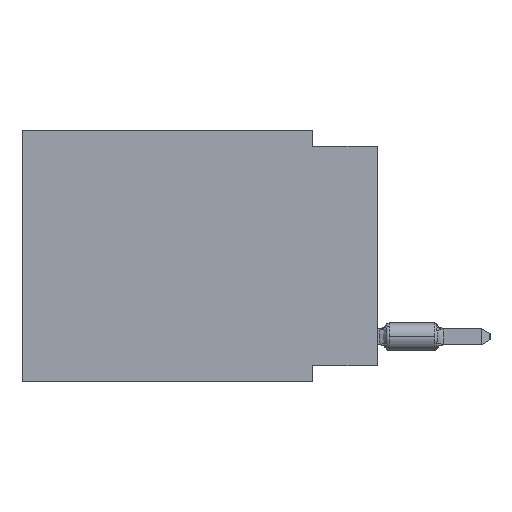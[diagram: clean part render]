
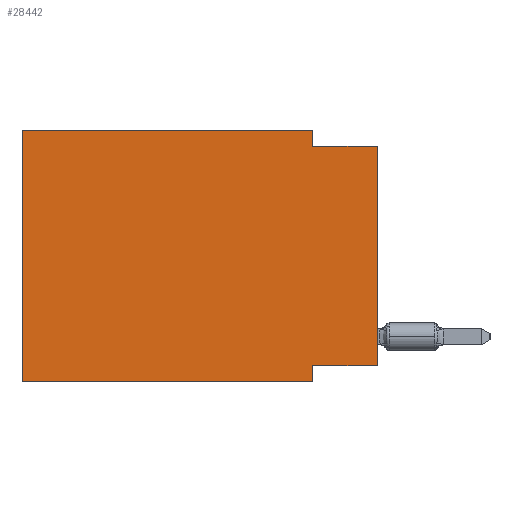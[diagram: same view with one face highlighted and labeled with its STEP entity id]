
A CAD part, left-side view. The second image highlights one B-rep face of the part: STEP entity #28442.
In plain terms, the highlighted planar face has unit normal (-1, 0, 0).
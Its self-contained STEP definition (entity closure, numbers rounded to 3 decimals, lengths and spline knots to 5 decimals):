
#246 = ORIENTED_EDGE ( 'NONE', *, *, #40371, .F. ) ;
#853 = DIRECTION ( 'NONE',  ( 0., -1., 0. ) ) ;
#866 = VERTEX_POINT ( 'NONE', #21386 ) ;
#4461 = LINE ( 'NONE', #12901, #59141 ) ;
#5445 = CARTESIAN_POINT ( 'NONE',  ( 0., 0.55, 0. ) ) ;
#7250 = CARTESIAN_POINT ( 'NONE',  ( 0., 0.1, -0.39 ) ) ;
#7344 = DIRECTION ( 'NONE',  ( 0., -1., 0. ) ) ;
#8345 = VERTEX_POINT ( 'NONE', #37222 ) ;
#8812 = EDGE_CURVE ( 'NONE', #8345, #47510, #38038, .T. ) ;
#9786 = DIRECTION ( 'NONE',  ( 0., 0., 1. ) ) ;
#10317 = VECTOR ( 'NONE', #9786, 39.37008 ) ;
#11092 = ORIENTED_EDGE ( 'NONE', *, *, #44853, .F. ) ;
#11502 = LINE ( 'NONE', #44207, #32913 ) ;
#12847 = VECTOR ( 'NONE', #15219, 39.37008 ) ;
#12901 = CARTESIAN_POINT ( 'NONE',  ( 0., 0.1, -0.39 ) ) ;
#13171 = ORIENTED_EDGE ( 'NONE', *, *, #41243, .F. ) ;
#13250 = VECTOR ( 'NONE', #52346, 39.37008 ) ;
#13631 = VECTOR ( 'NONE', #40186, 39.37008 ) ;
#14652 = CARTESIAN_POINT ( 'NONE',  ( 0., 0.1, 0. ) ) ;
#15219 = DIRECTION ( 'NONE',  ( 0., -1., 0. ) ) ;
#15557 = EDGE_LOOP ( 'NONE', ( #50107, #246, #11092, #27466, #23908, #59006, #13171, #59158 ) ) ;
#17220 = LINE ( 'NONE', #54148, #37976 ) ;
#20339 = CARTESIAN_POINT ( 'NONE',  ( 0., 0., -0.365 ) ) ;
#21386 = CARTESIAN_POINT ( 'NONE',  ( 0., 0.1, -0.025 ) ) ;
#23020 = PLANE ( 'NONE',  #30125 ) ;
#23908 = ORIENTED_EDGE ( 'NONE', *, *, #44401, .F. ) ;
#26352 = CARTESIAN_POINT ( 'NONE',  ( 0., 0., 0. ) ) ;
#27466 = ORIENTED_EDGE ( 'NONE', *, *, #31068, .F. ) ;
#27755 = VERTEX_POINT ( 'NONE', #30049 ) ;
#28442 = ADVANCED_FACE ( 'NONE', ( #37157 ), #23020, .F. ) ;
#29666 = CARTESIAN_POINT ( 'NONE',  ( 0., 0., -0.025 ) ) ;
#30049 = CARTESIAN_POINT ( 'NONE',  ( 0., 0.1, -0.365 ) ) ;
#30099 = DIRECTION ( 'NONE',  ( 0., 1., 0. ) ) ;
#30125 = AXIS2_PLACEMENT_3D ( 'NONE', #55450, #41665, #41961 ) ;
#31068 = EDGE_CURVE ( 'NONE', #32245, #34692, #33575, .T. ) ;
#31189 = VECTOR ( 'NONE', #853, 39.37008 ) ;
#31235 = VERTEX_POINT ( 'NONE', #29666 ) ;
#32245 = VERTEX_POINT ( 'NONE', #5445 ) ;
#32891 = DIRECTION ( 'NONE',  ( 0., 0., -1. ) ) ;
#32913 = VECTOR ( 'NONE', #30099, 39.37008 ) ;
#33575 = LINE ( 'NONE', #42006, #31189 ) ;
#33721 = CARTESIAN_POINT ( 'NONE',  ( 0., 0.1, 0. ) ) ;
#34692 = VERTEX_POINT ( 'NONE', #14652 ) ;
#36417 = VERTEX_POINT ( 'NONE', #20339 ) ;
#36528 = CARTESIAN_POINT ( 'NONE',  ( 0., 0.55, 0. ) ) ;
#37157 = FACE_OUTER_BOUND ( 'NONE', #15557, .T. ) ;
#37222 = CARTESIAN_POINT ( 'NONE',  ( 0., 0.55, -0.39 ) ) ;
#37240 = EDGE_CURVE ( 'NONE', #36417, #27755, #11502, .T. ) ;
#37941 = LINE ( 'NONE', #33721, #13250 ) ;
#37976 = VECTOR ( 'NONE', #7344, 39.37008 ) ;
#38038 = LINE ( 'NONE', #56344, #12847 ) ;
#40186 = DIRECTION ( 'NONE',  ( 0., 0., 1. ) ) ;
#40371 = EDGE_CURVE ( 'NONE', #866, #31235, #17220, .T. ) ;
#41045 = LINE ( 'NONE', #36528, #10317 ) ;
#41243 = EDGE_CURVE ( 'NONE', #27755, #47510, #4461, .T. ) ;
#41665 = DIRECTION ( 'NONE',  ( 1., 0., 0. ) ) ;
#41961 = DIRECTION ( 'NONE',  ( 0., 0., -1. ) ) ;
#42006 = CARTESIAN_POINT ( 'NONE',  ( 0., 0.55, 0. ) ) ;
#44207 = CARTESIAN_POINT ( 'NONE',  ( 0., 0., -0.365 ) ) ;
#44401 = EDGE_CURVE ( 'NONE', #8345, #32245, #41045, .T. ) ;
#44853 = EDGE_CURVE ( 'NONE', #34692, #866, #37941, .T. ) ;
#47510 = VERTEX_POINT ( 'NONE', #7250 ) ;
#48094 = EDGE_CURVE ( 'NONE', #36417, #31235, #53986, .T. ) ;
#50107 = ORIENTED_EDGE ( 'NONE', *, *, #48094, .T. ) ;
#52346 = DIRECTION ( 'NONE',  ( 0., 0., -1. ) ) ;
#53986 = LINE ( 'NONE', #26352, #13631 ) ;
#54148 = CARTESIAN_POINT ( 'NONE',  ( 0., 0., -0.025 ) ) ;
#55450 = CARTESIAN_POINT ( 'NONE',  ( 0., 0.55, 0. ) ) ;
#56344 = CARTESIAN_POINT ( 'NONE',  ( 0., 0.55, -0.39 ) ) ;
#59006 = ORIENTED_EDGE ( 'NONE', *, *, #8812, .T. ) ;
#59141 = VECTOR ( 'NONE', #32891, 39.37008 ) ;
#59158 = ORIENTED_EDGE ( 'NONE', *, *, #37240, .F. ) ;
